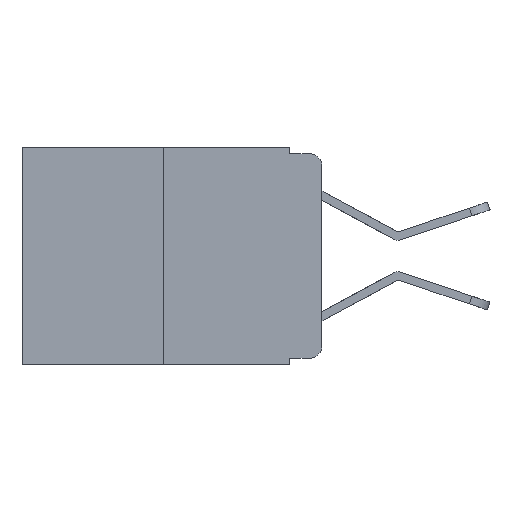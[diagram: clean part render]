
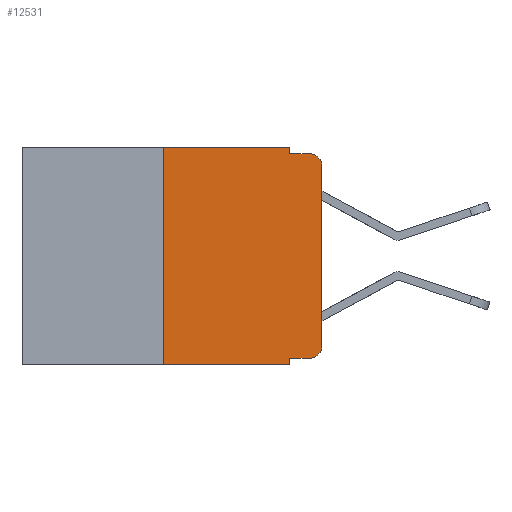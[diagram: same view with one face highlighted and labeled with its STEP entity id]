
A CAD part, left-side view. The second image highlights one B-rep face of the part: STEP entity #12531.
In plain terms, the highlighted planar face has unit normal (-1, 0, 0).
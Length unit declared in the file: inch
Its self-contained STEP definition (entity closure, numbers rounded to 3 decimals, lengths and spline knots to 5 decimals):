
#9 = DIRECTION ( 'NONE',  ( -1., 0., 0. ) ) ;
#118 = DIRECTION ( 'NONE',  ( -1., 0., 0. ) ) ;
#439 = VECTOR ( 'NONE', #5765, 39.37008 ) ;
#467 = CARTESIAN_POINT ( 'NONE',  ( 0., 0.473, 0. ) ) ;
#501 = VERTEX_POINT ( 'NONE', #4575 ) ;
#581 = EDGE_CURVE ( 'NONE', #7860, #501, #9584, .T. ) ;
#855 = ORIENTED_EDGE ( 'NONE', *, *, #6013, .F. ) ;
#911 = EDGE_CURVE ( 'NONE', #3080, #3600, #14581, .T. ) ;
#1395 = LINE ( 'NONE', #467, #13888 ) ;
#1604 = CARTESIAN_POINT ( 'NONE',  ( 0., 0.051, 0. ) ) ;
#1738 = CARTESIAN_POINT ( 'NONE',  ( 0., 0., 0. ) ) ;
#1785 = DIRECTION ( 'NONE',  ( 0., 0., 1. ) ) ;
#1816 = CARTESIAN_POINT ( 'NONE',  ( 0., 0.25, -0.343 ) ) ;
#1968 = CARTESIAN_POINT ( 'NONE',  ( 0., 0.051, 0. ) ) ;
#2016 = ORIENTED_EDGE ( 'NONE', *, *, #10635, .T. ) ;
#2292 = ORIENTED_EDGE ( 'NONE', *, *, #911, .T. ) ;
#2370 = EDGE_CURVE ( 'NONE', #3600, #10148, #5892, .T. ) ;
#2522 = CARTESIAN_POINT ( 'NONE',  ( 0., 0.473, -0.343 ) ) ;
#2625 = CARTESIAN_POINT ( 'NONE',  ( 0., 0.051, -0.01 ) ) ;
#2697 = EDGE_CURVE ( 'NONE', #3722, #3080, #5180, .T. ) ;
#3080 = VERTEX_POINT ( 'NONE', #9146 ) ;
#3093 = EDGE_LOOP ( 'NONE', ( #11196, #2016, #3931, #14760, #10065, #10328, #13389, #855, #14988, #2292 ) ) ;
#3290 = PLANE ( 'NONE',  #4998 ) ;
#3545 = LINE ( 'NONE', #1604, #439 ) ;
#3600 = VERTEX_POINT ( 'NONE', #13918 ) ;
#3722 = VERTEX_POINT ( 'NONE', #11696 ) ;
#3931 = ORIENTED_EDGE ( 'NONE', *, *, #581, .F. ) ;
#4040 = VERTEX_POINT ( 'NONE', #1816 ) ;
#4468 = VERTEX_POINT ( 'NONE', #4641 ) ;
#4546 = DIRECTION ( 'NONE',  ( 1., 0., 0. ) ) ;
#4575 = CARTESIAN_POINT ( 'NONE',  ( 0., 0.02, -0.01 ) ) ;
#4641 = CARTESIAN_POINT ( 'NONE',  ( 0., 0.051, -0.343 ) ) ;
#4998 = AXIS2_PLACEMENT_3D ( 'NONE', #11459, #4546, #12572 ) ;
#5020 = VECTOR ( 'NONE', #12837, 39.37008 ) ;
#5180 = LINE ( 'NONE', #8712, #13853 ) ;
#5197 = DIRECTION ( 'NONE',  ( 0., -1., 0. ) ) ;
#5235 = VECTOR ( 'NONE', #13026, 39.37008 ) ;
#5765 = DIRECTION ( 'NONE',  ( 0., 0., -1. ) ) ;
#5892 = LINE ( 'NONE', #1738, #14871 ) ;
#6013 = EDGE_CURVE ( 'NONE', #3722, #4468, #11140, .T. ) ;
#6232 = AXIS2_PLACEMENT_3D ( 'NONE', #8334, #9, #9102 ) ;
#6441 = CARTESIAN_POINT ( 'NONE',  ( 0., 0., -0.03 ) ) ;
#6475 = VECTOR ( 'NONE', #14217, 39.37008 ) ;
#7527 = LINE ( 'NONE', #13962, #13128 ) ;
#7584 = EDGE_CURVE ( 'NONE', #4040, #11579, #7527, .T. ) ;
#7619 = CARTESIAN_POINT ( 'NONE',  ( 0., 0.02, -0.03 ) ) ;
#7860 = VERTEX_POINT ( 'NONE', #2625 ) ;
#8270 = CARTESIAN_POINT ( 'NONE',  ( 0., 0.051, 0. ) ) ;
#8334 = CARTESIAN_POINT ( 'NONE',  ( 0., 0.02, -0.313 ) ) ;
#8712 = CARTESIAN_POINT ( 'NONE',  ( 0., 0.051, -0.333 ) ) ;
#8751 = CARTESIAN_POINT ( 'NONE',  ( 0., 0.051, -0.01 ) ) ;
#8769 = DIRECTION ( 'NONE',  ( 0., 0., -1. ) ) ;
#9078 = DIRECTION ( 'NONE',  ( 0., -1., 0. ) ) ;
#9102 = DIRECTION ( 'NONE',  ( 0., 0., -1. ) ) ;
#9133 = EDGE_CURVE ( 'NONE', #11436, #7860, #3545, .T. ) ;
#9146 = CARTESIAN_POINT ( 'NONE',  ( 0., 0.02, -0.333 ) ) ;
#9584 = LINE ( 'NONE', #8751, #6475 ) ;
#10065 = ORIENTED_EDGE ( 'NONE', *, *, #13014, .F. ) ;
#10148 = VERTEX_POINT ( 'NONE', #6441 ) ;
#10328 = ORIENTED_EDGE ( 'NONE', *, *, #7584, .F. ) ;
#10635 = EDGE_CURVE ( 'NONE', #10148, #501, #15100, .T. ) ;
#11140 = LINE ( 'NONE', #1968, #5020 ) ;
#11196 = ORIENTED_EDGE ( 'NONE', *, *, #2370, .T. ) ;
#11436 = VERTEX_POINT ( 'NONE', #8270 ) ;
#11459 = CARTESIAN_POINT ( 'NONE',  ( 0., 0.473, 0. ) ) ;
#11579 = VERTEX_POINT ( 'NONE', #14049 ) ;
#11696 = CARTESIAN_POINT ( 'NONE',  ( 0., 0.051, -0.333 ) ) ;
#12177 = EDGE_CURVE ( 'NONE', #4040, #4468, #14249, .T. ) ;
#12531 = ADVANCED_FACE ( 'NONE', ( #12724 ), #3290, .F. ) ;
#12572 = DIRECTION ( 'NONE',  ( 0., 0., -1. ) ) ;
#12724 = FACE_OUTER_BOUND ( 'NONE', #3093, .T. ) ;
#12837 = DIRECTION ( 'NONE',  ( 0., 0., -1. ) ) ;
#13014 = EDGE_CURVE ( 'NONE', #11579, #11436, #1395, .T. ) ;
#13026 = DIRECTION ( 'NONE',  ( 0., -1., 0. ) ) ;
#13128 = VECTOR ( 'NONE', #13680, 39.37008 ) ;
#13341 = AXIS2_PLACEMENT_3D ( 'NONE', #7619, #118, #8769 ) ;
#13389 = ORIENTED_EDGE ( 'NONE', *, *, #12177, .T. ) ;
#13680 = DIRECTION ( 'NONE',  ( 0., 0., 1. ) ) ;
#13853 = VECTOR ( 'NONE', #5197, 39.37008 ) ;
#13888 = VECTOR ( 'NONE', #9078, 39.37008 ) ;
#13918 = CARTESIAN_POINT ( 'NONE',  ( 0., 0., -0.313 ) ) ;
#13962 = CARTESIAN_POINT ( 'NONE',  ( 0., 0.25, 0. ) ) ;
#14049 = CARTESIAN_POINT ( 'NONE',  ( 0., 0.25, 0. ) ) ;
#14217 = DIRECTION ( 'NONE',  ( 0., -1., 0. ) ) ;
#14249 = LINE ( 'NONE', #2522, #5235 ) ;
#14581 = CIRCLE ( 'NONE', #6232, 0.02 ) ;
#14760 = ORIENTED_EDGE ( 'NONE', *, *, #9133, .F. ) ;
#14871 = VECTOR ( 'NONE', #1785, 39.37008 ) ;
#14988 = ORIENTED_EDGE ( 'NONE', *, *, #2697, .T. ) ;
#15100 = CIRCLE ( 'NONE', #13341, 0.02 ) ;
